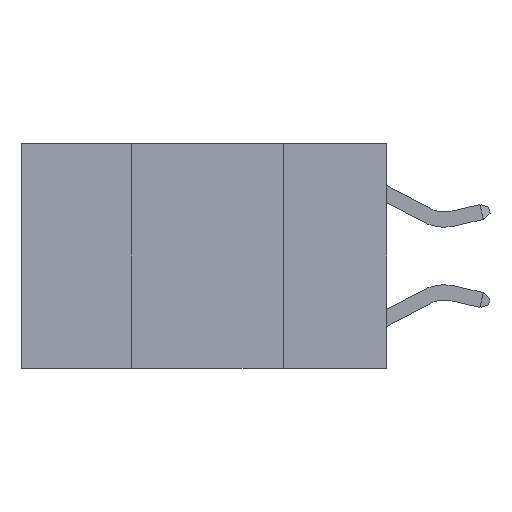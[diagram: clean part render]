
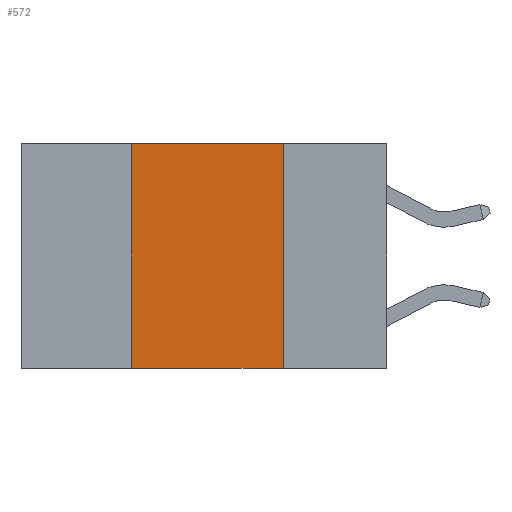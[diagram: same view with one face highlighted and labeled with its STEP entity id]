
A CAD part, left-side view. The second image highlights one B-rep face of the part: STEP entity #572.
In plain terms, the highlighted planar face has unit normal (-1, 0, 0).
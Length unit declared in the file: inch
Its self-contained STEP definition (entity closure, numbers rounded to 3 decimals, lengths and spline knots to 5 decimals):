
#194 = CARTESIAN_POINT ( 'NONE',  ( 0., 0.6, -0.37 ) ) ;
#332 = EDGE_CURVE ( 'NONE', #6674, #7690, #795, .T. ) ;
#513 = PLANE ( 'NONE',  #8975 ) ;
#572 = ADVANCED_FACE ( 'NONE', ( #2000 ), #513, .F. ) ;
#795 = LINE ( 'NONE', #194, #6598 ) ;
#916 = CARTESIAN_POINT ( 'NONE',  ( 0., 0.6, 0. ) ) ;
#1001 = EDGE_CURVE ( 'NONE', #6674, #4741, #4092, .T. ) ;
#1019 = EDGE_CURVE ( 'NONE', #8303, #7690, #7697, .T. ) ;
#1247 = CARTESIAN_POINT ( 'NONE',  ( 0., 0.42, 0. ) ) ;
#1347 = ORIENTED_EDGE ( 'NONE', *, *, #1019, .F. ) ;
#1783 = DIRECTION ( 'NONE',  ( 1., 0., 0. ) ) ;
#1989 = VECTOR ( 'NONE', #9493, 39.37008 ) ;
#2000 = FACE_OUTER_BOUND ( 'NONE', #9759, .T. ) ;
#2445 = DIRECTION ( 'NONE',  ( 0., 0., -1. ) ) ;
#2692 = CARTESIAN_POINT ( 'NONE',  ( 0., 0.6, 0. ) ) ;
#3379 = VECTOR ( 'NONE', #5688, 39.37008 ) ;
#3515 = CARTESIAN_POINT ( 'NONE',  ( 0., 0.42, -0.37 ) ) ;
#3784 = ORIENTED_EDGE ( 'NONE', *, *, #332, .T. ) ;
#4092 = LINE ( 'NONE', #1247, #1989 ) ;
#4167 = EDGE_CURVE ( 'NONE', #4741, #8303, #7488, .T. ) ;
#4607 = CARTESIAN_POINT ( 'NONE',  ( 0., 0.17, -0.37 ) ) ;
#4741 = VERTEX_POINT ( 'NONE', #6953 ) ;
#5263 = CARTESIAN_POINT ( 'NONE',  ( 0., 0.17, 0. ) ) ;
#5688 = DIRECTION ( 'NONE',  ( 0., -1., 0. ) ) ;
#6027 = DIRECTION ( 'NONE',  ( 0., -1., 0. ) ) ;
#6477 = ORIENTED_EDGE ( 'NONE', *, *, #4167, .F. ) ;
#6598 = VECTOR ( 'NONE', #6027, 39.37008 ) ;
#6674 = VERTEX_POINT ( 'NONE', #3515 ) ;
#6953 = CARTESIAN_POINT ( 'NONE',  ( 0., 0.42, 0. ) ) ;
#7488 = LINE ( 'NONE', #916, #3379 ) ;
#7690 = VERTEX_POINT ( 'NONE', #4607 ) ;
#7697 = LINE ( 'NONE', #9158, #9694 ) ;
#7982 = ORIENTED_EDGE ( 'NONE', *, *, #1001, .F. ) ;
#8303 = VERTEX_POINT ( 'NONE', #5263 ) ;
#8975 = AXIS2_PLACEMENT_3D ( 'NONE', #2692, #1783, #2445 ) ;
#9158 = CARTESIAN_POINT ( 'NONE',  ( 0., 0.17, 0. ) ) ;
#9493 = DIRECTION ( 'NONE',  ( 0., 0., 1. ) ) ;
#9694 = VECTOR ( 'NONE', #9790, 39.37008 ) ;
#9759 = EDGE_LOOP ( 'NONE', ( #1347, #6477, #7982, #3784 ) ) ;
#9790 = DIRECTION ( 'NONE',  ( 0., 0., -1. ) ) ;
